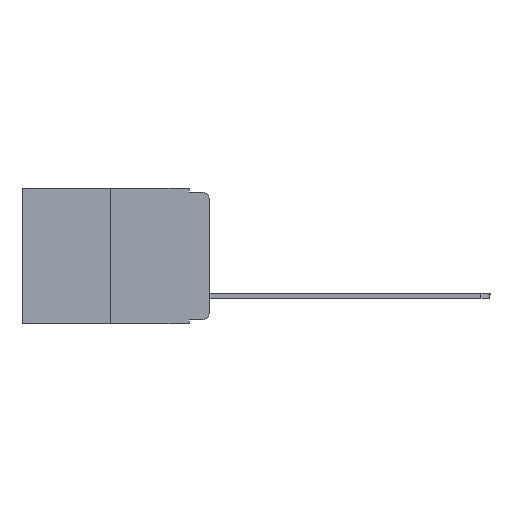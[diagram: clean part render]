
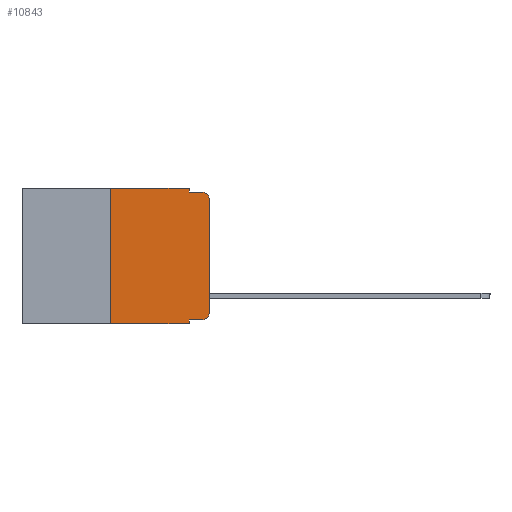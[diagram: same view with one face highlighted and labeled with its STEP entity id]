
A CAD part, left-side view. The second image highlights one B-rep face of the part: STEP entity #10843.
In plain terms, the highlighted planar face has unit normal (-1, 0, 0).
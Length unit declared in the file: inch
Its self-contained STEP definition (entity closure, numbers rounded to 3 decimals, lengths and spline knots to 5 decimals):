
#70 = VERTEX_POINT ( 'NONE', #8537 ) ;
#73 = ORIENTED_EDGE ( 'NONE', *, *, #5238, .F. ) ;
#371 = EDGE_CURVE ( 'NONE', #9227, #4781, #8994, .T. ) ;
#376 = CARTESIAN_POINT ( 'NONE',  ( 0., 0.25, -0.343 ) ) ;
#391 = FACE_OUTER_BOUND ( 'NONE', #9245, .T. ) ;
#501 = ORIENTED_EDGE ( 'NONE', *, *, #10672, .T. ) ;
#576 = EDGE_CURVE ( 'NONE', #5322, #9837, #3423, .T. ) ;
#1430 = VERTEX_POINT ( 'NONE', #376 ) ;
#1465 = CARTESIAN_POINT ( 'NONE',  ( 0., 0.051, -0.333 ) ) ;
#1630 = DIRECTION ( 'NONE',  ( 0., -1., 0. ) ) ;
#1647 = AXIS2_PLACEMENT_3D ( 'NONE', #7262, #9224, #12082 ) ;
#1699 = CARTESIAN_POINT ( 'NONE',  ( 0., 0.473, 0. ) ) ;
#1711 = ORIENTED_EDGE ( 'NONE', *, *, #9054, .T. ) ;
#1976 = ORIENTED_EDGE ( 'NONE', *, *, #10268, .F. ) ;
#2140 = EDGE_CURVE ( 'NONE', #1430, #5388, #7517, .T. ) ;
#2176 = EDGE_CURVE ( 'NONE', #10491, #5322, #4910, .T. ) ;
#2187 = CARTESIAN_POINT ( 'NONE',  ( 0., 0.473, 0. ) ) ;
#2341 = ORIENTED_EDGE ( 'NONE', *, *, #2140, .F. ) ;
#2671 = VECTOR ( 'NONE', #9972, 39.37008 ) ;
#2674 = CARTESIAN_POINT ( 'NONE',  ( 0., 0.02, -0.01 ) ) ;
#2963 = ORIENTED_EDGE ( 'NONE', *, *, #9347, .F. ) ;
#3068 = CARTESIAN_POINT ( 'NONE',  ( 0., 0., 0. ) ) ;
#3119 = DIRECTION ( 'NONE',  ( 1., 0., 0. ) ) ;
#3136 = CARTESIAN_POINT ( 'NONE',  ( 0., 0., -0.313 ) ) ;
#3214 = CIRCLE ( 'NONE', #10319, 0.02 ) ;
#3311 = VECTOR ( 'NONE', #5882, 39.37008 ) ;
#3423 = CIRCLE ( 'NONE', #1647, 0.02 ) ;
#3565 = CARTESIAN_POINT ( 'NONE',  ( 0., 0.473, -0.343 ) ) ;
#3869 = ORIENTED_EDGE ( 'NONE', *, *, #8395, .F. ) ;
#3971 = ORIENTED_EDGE ( 'NONE', *, *, #371, .T. ) ;
#4038 = ORIENTED_EDGE ( 'NONE', *, *, #576, .T. ) ;
#4259 = VECTOR ( 'NONE', #1630, 39.37008 ) ;
#4278 = PLANE ( 'NONE',  #9775 ) ;
#4781 = VERTEX_POINT ( 'NONE', #10813 ) ;
#4910 = LINE ( 'NONE', #3068, #12057 ) ;
#4912 = CARTESIAN_POINT ( 'NONE',  ( 0., 0.051, 0. ) ) ;
#5177 = VECTOR ( 'NONE', #7638, 39.37008 ) ;
#5204 = DIRECTION ( 'NONE',  ( 0., 0., -1. ) ) ;
#5238 = EDGE_CURVE ( 'NONE', #12092, #9837, #10733, .T. ) ;
#5322 = VERTEX_POINT ( 'NONE', #5461 ) ;
#5388 = VERTEX_POINT ( 'NONE', #11044 ) ;
#5395 = LINE ( 'NONE', #6207, #2671 ) ;
#5461 = CARTESIAN_POINT ( 'NONE',  ( 0., 0., -0.03 ) ) ;
#5826 = VECTOR ( 'NONE', #6536, 39.37008 ) ;
#5834 = CARTESIAN_POINT ( 'NONE',  ( 0., 0.02, -0.313 ) ) ;
#5882 = DIRECTION ( 'NONE',  ( 0., -1., 0. ) ) ;
#6027 = DIRECTION ( 'NONE',  ( 0., 0., 1. ) ) ;
#6207 = CARTESIAN_POINT ( 'NONE',  ( 0., 0.051, 0. ) ) ;
#6536 = DIRECTION ( 'NONE',  ( 0., -1., 0. ) ) ;
#6559 = ORIENTED_EDGE ( 'NONE', *, *, #2176, .T. ) ;
#6741 = VECTOR ( 'NONE', #8790, 39.37008 ) ;
#7033 = DIRECTION ( 'NONE',  ( 0., 0., 1. ) ) ;
#7262 = CARTESIAN_POINT ( 'NONE',  ( 0., 0.02, -0.03 ) ) ;
#7517 = LINE ( 'NONE', #11313, #11847 ) ;
#7638 = DIRECTION ( 'NONE',  ( 0., 0., -1. ) ) ;
#8395 = EDGE_CURVE ( 'NONE', #70, #12092, #5395, .T. ) ;
#8537 = CARTESIAN_POINT ( 'NONE',  ( 0., 0.051, 0. ) ) ;
#8739 = LINE ( 'NONE', #4912, #5177 ) ;
#8790 = DIRECTION ( 'NONE',  ( 0., -1., 0. ) ) ;
#8994 = LINE ( 'NONE', #1465, #3311 ) ;
#9054 = EDGE_CURVE ( 'NONE', #1430, #9864, #10188, .T. ) ;
#9097 = LINE ( 'NONE', #1699, #4259 ) ;
#9224 = DIRECTION ( 'NONE',  ( -1., 0., 0. ) ) ;
#9227 = VERTEX_POINT ( 'NONE', #10739 ) ;
#9245 = EDGE_LOOP ( 'NONE', ( #6559, #4038, #73, #3869, #2963, #2341, #1711, #1976, #3971, #501 ) ) ;
#9347 = EDGE_CURVE ( 'NONE', #5388, #70, #9097, .T. ) ;
#9564 = CARTESIAN_POINT ( 'NONE',  ( 0., 0.051, -0.343 ) ) ;
#9662 = DIRECTION ( 'NONE',  ( -1., 0., 0. ) ) ;
#9665 = CARTESIAN_POINT ( 'NONE',  ( 0., 0.051, -0.01 ) ) ;
#9775 = AXIS2_PLACEMENT_3D ( 'NONE', #2187, #3119, #5204 ) ;
#9837 = VERTEX_POINT ( 'NONE', #2674 ) ;
#9864 = VERTEX_POINT ( 'NONE', #9564 ) ;
#9972 = DIRECTION ( 'NONE',  ( 0., 0., -1. ) ) ;
#10188 = LINE ( 'NONE', #3565, #5826 ) ;
#10268 = EDGE_CURVE ( 'NONE', #9227, #9864, #8739, .T. ) ;
#10319 = AXIS2_PLACEMENT_3D ( 'NONE', #5834, #9662, #10352 ) ;
#10352 = DIRECTION ( 'NONE',  ( 0., 0., -1. ) ) ;
#10491 = VERTEX_POINT ( 'NONE', #3136 ) ;
#10672 = EDGE_CURVE ( 'NONE', #4781, #10491, #3214, .T. ) ;
#10733 = LINE ( 'NONE', #10796, #6741 ) ;
#10739 = CARTESIAN_POINT ( 'NONE',  ( 0., 0.051, -0.333 ) ) ;
#10796 = CARTESIAN_POINT ( 'NONE',  ( 0., 0.051, -0.01 ) ) ;
#10813 = CARTESIAN_POINT ( 'NONE',  ( 0., 0.02, -0.333 ) ) ;
#10843 = ADVANCED_FACE ( 'NONE', ( #391 ), #4278, .F. ) ;
#11044 = CARTESIAN_POINT ( 'NONE',  ( 0., 0.25, 0. ) ) ;
#11313 = CARTESIAN_POINT ( 'NONE',  ( 0., 0.25, 0. ) ) ;
#11847 = VECTOR ( 'NONE', #6027, 39.37008 ) ;
#12057 = VECTOR ( 'NONE', #7033, 39.37008 ) ;
#12082 = DIRECTION ( 'NONE',  ( 0., 0., -1. ) ) ;
#12092 = VERTEX_POINT ( 'NONE', #9665 ) ;
